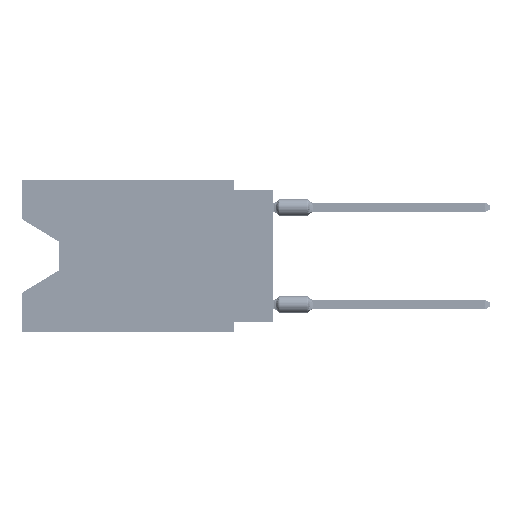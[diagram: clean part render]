
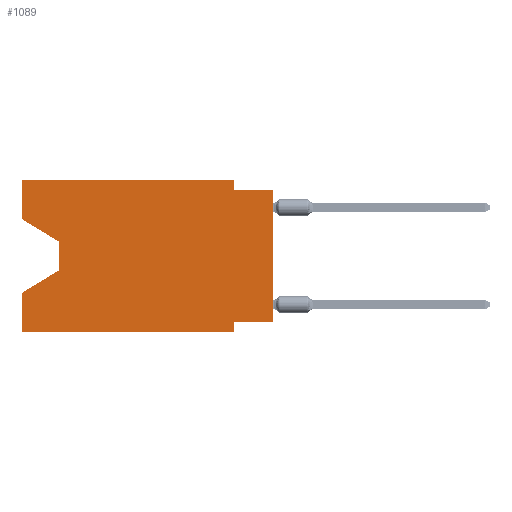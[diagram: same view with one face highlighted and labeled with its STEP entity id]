
A CAD part, left-side view. The second image highlights one B-rep face of the part: STEP entity #1089.
In plain terms, the highlighted planar face has unit normal (-1, 0, 0).
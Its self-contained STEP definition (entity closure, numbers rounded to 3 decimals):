
#219 = CARTESIAN_POINT ( 'NONE',  ( 0., 2.54, -0.635 ) ) ;
#228 = CARTESIAN_POINT ( 'NONE',  ( 0., 0., -0.635 ) ) ;
#563 = LINE ( 'NONE', #68374, #13102 ) ;
#1089 = ADVANCED_FACE ( 'NONE', ( #29467 ), #35444, .F. ) ;
#1748 = DIRECTION ( 'NONE',  ( 0., 0., 1. ) ) ;
#2052 = CARTESIAN_POINT ( 'NONE',  ( 0., 16.383, -9.906 ) ) ;
#4204 = DIRECTION ( 'NONE',  ( 0., -1., 0. ) ) ;
#6078 = CARTESIAN_POINT ( 'NONE',  ( 0., 16.383, 0. ) ) ;
#7606 = CARTESIAN_POINT ( 'NONE',  ( 0., 16.383, -9.906 ) ) ;
#8920 = ORIENTED_EDGE ( 'NONE', *, *, #74747, .F. ) ;
#9040 = EDGE_CURVE ( 'NONE', #10076, #54182, #71354, .T. ) ;
#9483 = CARTESIAN_POINT ( 'NONE',  ( 0., 16.383, -7.36 ) ) ;
#10076 = VERTEX_POINT ( 'NONE', #37740 ) ;
#10584 = LINE ( 'NONE', #76432, #29364 ) ;
#10704 = CARTESIAN_POINT ( 'NONE',  ( 0., 2.54, -9.906 ) ) ;
#10981 = ORIENTED_EDGE ( 'NONE', *, *, #29637, .T. ) ;
#11129 = VECTOR ( 'NONE', #61109, 1000. ) ;
#11526 = CARTESIAN_POINT ( 'NONE',  ( 0., 16.383, 0. ) ) ;
#13102 = VECTOR ( 'NONE', #1748, 1000. ) ;
#13239 = DIRECTION ( 'NONE',  ( 0., -1., 0. ) ) ;
#15046 = ORIENTED_EDGE ( 'NONE', *, *, #55833, .F. ) ;
#16106 = CARTESIAN_POINT ( 'NONE',  ( 0., 0., 0. ) ) ;
#16125 = EDGE_CURVE ( 'NONE', #64832, #63069, #60173, .T. ) ;
#16421 = ORIENTED_EDGE ( 'NONE', *, *, #19009, .F. ) ;
#18861 = DIRECTION ( 'NONE',  ( 0., 0., 1. ) ) ;
#19009 = EDGE_CURVE ( 'NONE', #56704, #72136, #36002, .T. ) ;
#20224 = VERTEX_POINT ( 'NONE', #55174 ) ;
#20781 = EDGE_LOOP ( 'NONE', ( #49422, #29855, #10981, #73004, #59888, #15046, #62589, #56502, #64068, #60705, #8920, #16421 ) ) ;
#20791 = VECTOR ( 'NONE', #72815, 1000. ) ;
#21622 = EDGE_CURVE ( 'NONE', #43858, #31698, #21657, .T. ) ;
#21657 = LINE ( 'NONE', #39590, #77414 ) ;
#21905 = VERTEX_POINT ( 'NONE', #9483 ) ;
#24550 = CARTESIAN_POINT ( 'NONE',  ( 0., 0., -9.271 ) ) ;
#25519 = CARTESIAN_POINT ( 'NONE',  ( 0., 2.54, 0. ) ) ;
#25885 = DIRECTION ( 'NONE',  ( 0., 0.855, -0.519 ) ) ;
#27479 = DIRECTION ( 'NONE',  ( 0., 0., -1. ) ) ;
#29364 = VECTOR ( 'NONE', #4204, 1000. ) ;
#29467 = FACE_OUTER_BOUND ( 'NONE', #20781, .T. ) ;
#29637 = EDGE_CURVE ( 'NONE', #54182, #21905, #60593, .T. ) ;
#29846 = DIRECTION ( 'NONE',  ( 0., 0., -1. ) ) ;
#29850 = CARTESIAN_POINT ( 'NONE',  ( 0., 0., -9.271 ) ) ;
#29855 = ORIENTED_EDGE ( 'NONE', *, *, #9040, .T. ) ;
#30647 = DIRECTION ( 'NONE',  ( 1., 0., 0. ) ) ;
#31698 = VERTEX_POINT ( 'NONE', #219 ) ;
#33122 = CARTESIAN_POINT ( 'NONE',  ( 0., 2.54, -9.271 ) ) ;
#35444 = PLANE ( 'NONE',  #42263 ) ;
#36002 = LINE ( 'NONE', #66713, #62046 ) ;
#36768 = CARTESIAN_POINT ( 'NONE',  ( 0., 16.383, -2.546 ) ) ;
#37157 = LINE ( 'NONE', #2052, #72098 ) ;
#37454 = EDGE_CURVE ( 'NONE', #65202, #20224, #37157, .T. ) ;
#37740 = CARTESIAN_POINT ( 'NONE',  ( 0., 13.97, -4.013 ) ) ;
#38175 = VECTOR ( 'NONE', #39454, 1000. ) ;
#39454 = DIRECTION ( 'NONE',  ( 0., 0., -1. ) ) ;
#39590 = CARTESIAN_POINT ( 'NONE',  ( 0., 2.54, 0. ) ) ;
#41001 = LINE ( 'NONE', #10704, #38175 ) ;
#42243 = CARTESIAN_POINT ( 'NONE',  ( 0., 13.97, -5.893 ) ) ;
#42263 = AXIS2_PLACEMENT_3D ( 'NONE', #11526, #30647, #29846 ) ;
#42942 = VECTOR ( 'NONE', #27479, 1000. ) ;
#43858 = VERTEX_POINT ( 'NONE', #25519 ) ;
#45575 = DIRECTION ( 'NONE',  ( 0., 0., -1. ) ) ;
#46280 = CARTESIAN_POINT ( 'NONE',  ( 0., 13.97, -5.893 ) ) ;
#47355 = EDGE_CURVE ( 'NONE', #31698, #55163, #10584, .T. ) ;
#47666 = CARTESIAN_POINT ( 'NONE',  ( 0., 16.383, 0. ) ) ;
#49121 = LINE ( 'NONE', #36768, #11129 ) ;
#49422 = ORIENTED_EDGE ( 'NONE', *, *, #52752, .T. ) ;
#52752 = EDGE_CURVE ( 'NONE', #56704, #10076, #49121, .T. ) ;
#54182 = VERTEX_POINT ( 'NONE', #46280 ) ;
#55163 = VERTEX_POINT ( 'NONE', #228 ) ;
#55174 = CARTESIAN_POINT ( 'NONE',  ( 0., 2.54, -9.906 ) ) ;
#55833 = EDGE_CURVE ( 'NONE', #63069, #20224, #41001, .T. ) ;
#56502 = ORIENTED_EDGE ( 'NONE', *, *, #67278, .T. ) ;
#56704 = VERTEX_POINT ( 'NONE', #66633 ) ;
#58185 = CARTESIAN_POINT ( 'NONE',  ( 0., 13.97, -4.013 ) ) ;
#59794 = DIRECTION ( 'NONE',  ( 0., 1., 0. ) ) ;
#59888 = ORIENTED_EDGE ( 'NONE', *, *, #37454, .T. ) ;
#60173 = LINE ( 'NONE', #29850, #73058 ) ;
#60593 = LINE ( 'NONE', #42243, #67079 ) ;
#60705 = ORIENTED_EDGE ( 'NONE', *, *, #21622, .F. ) ;
#61109 = DIRECTION ( 'NONE',  ( 0., -0.855, -0.519 ) ) ;
#62046 = VECTOR ( 'NONE', #18861, 1000. ) ;
#62589 = ORIENTED_EDGE ( 'NONE', *, *, #16125, .F. ) ;
#63069 = VERTEX_POINT ( 'NONE', #33122 ) ;
#64068 = ORIENTED_EDGE ( 'NONE', *, *, #47355, .F. ) ;
#64832 = VERTEX_POINT ( 'NONE', #24550 ) ;
#65202 = VERTEX_POINT ( 'NONE', #7606 ) ;
#65243 = LINE ( 'NONE', #47666, #20791 ) ;
#66633 = CARTESIAN_POINT ( 'NONE',  ( 0., 16.383, -2.546 ) ) ;
#66713 = CARTESIAN_POINT ( 'NONE',  ( 0., 16.383, 0. ) ) ;
#67079 = VECTOR ( 'NONE', #25885, 1000. ) ;
#67278 = EDGE_CURVE ( 'NONE', #64832, #55163, #74882, .T. ) ;
#67612 = VECTOR ( 'NONE', #68497, 1000. ) ;
#68374 = CARTESIAN_POINT ( 'NONE',  ( 0., 16.383, 0. ) ) ;
#68497 = DIRECTION ( 'NONE',  ( 0., 0., 1. ) ) ;
#70092 = EDGE_CURVE ( 'NONE', #65202, #21905, #563, .T. ) ;
#71354 = LINE ( 'NONE', #58185, #42942 ) ;
#72098 = VECTOR ( 'NONE', #13239, 1000. ) ;
#72136 = VERTEX_POINT ( 'NONE', #6078 ) ;
#72815 = DIRECTION ( 'NONE',  ( 0., -1., 0. ) ) ;
#73004 = ORIENTED_EDGE ( 'NONE', *, *, #70092, .F. ) ;
#73058 = VECTOR ( 'NONE', #59794, 1000. ) ;
#74747 = EDGE_CURVE ( 'NONE', #72136, #43858, #65243, .T. ) ;
#74882 = LINE ( 'NONE', #16106, #67612 ) ;
#76432 = CARTESIAN_POINT ( 'NONE',  ( 0., 0., -0.635 ) ) ;
#77414 = VECTOR ( 'NONE', #45575, 1000. ) ;
